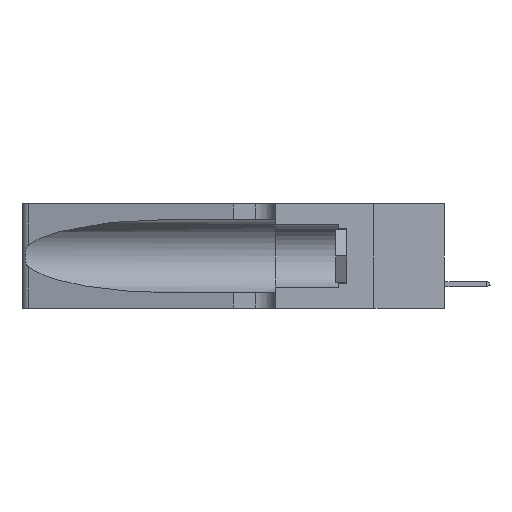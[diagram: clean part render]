
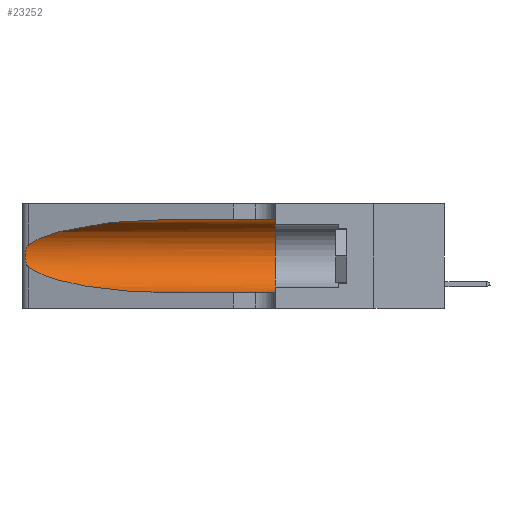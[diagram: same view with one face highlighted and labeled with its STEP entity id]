
A CAD part, left-side view. The second image highlights one B-rep face of the part: STEP entity #23252.
In plain terms, the highlighted cylindrical face has radius 3.308 mm (diameter 6.617 mm), a partial arc.
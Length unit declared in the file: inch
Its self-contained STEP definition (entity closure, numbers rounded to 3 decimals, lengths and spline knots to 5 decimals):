
#1957 = VERTEX_POINT ( 'NONE', #3929 ) ;
#2372 = CARTESIAN_POINT ( 'NONE',  ( 0.1305, 0.35, 0.05475 ) ) ;
#2921 = ORIENTED_EDGE ( 'NONE', *, *, #27712, .T. ) ;
#3313 = FACE_OUTER_BOUND ( 'NONE', #23588, .T. ) ;
#3369 = ORIENTED_EDGE ( 'NONE', *, *, #18472, .T. ) ;
#3929 = CARTESIAN_POINT ( 'NONE',  ( 0.1305, 0.35, 0.31525 ) ) ;
#4199 = CARTESIAN_POINT ( 'NONE',  ( 0.26018, 1.23835, 0.19895 ) ) ;
#4342 = CARTESIAN_POINT ( 'NONE',  ( 0.25854, 1.2359, 0.20912 ) ) ;
#6257 =( BOUNDED_CURVE ( )  B_SPLINE_CURVE ( 3, ( #7449, #13688, #25617, #22827 ),
 .UNSPECIFIED., .F., .T. ) 
 B_SPLINE_CURVE_WITH_KNOTS ( ( 4, 4 ),
 ( 3.44316, 4.71239 ),
 .UNSPECIFIED. ) 
 CURVE ( )  GEOMETRIC_REPRESENTATION_ITEM ( )  RATIONAL_B_SPLINE_CURVE ( ( 1., 0.87, 0.87, 1. ) ) 
 REPRESENTATION_ITEM ( '' )  );
#6865 = EDGE_CURVE ( 'NONE', #1957, #12653, #11539, .T. ) ;
#7319 = CARTESIAN_POINT ( 'NONE',  ( 0.26075, 1.23896, 0.178 ) ) ;
#7449 = CARTESIAN_POINT ( 'NONE',  ( 0.25487, 1.22718, 0.14631 ) ) ;
#9013 = CARTESIAN_POINT ( 'NONE',  ( 0.18966, 0.96281, 0.31525 ) ) ;
#10514 = CARTESIAN_POINT ( 'NONE',  ( 0.26017, 1.23833, 0.17102 ) ) ;
#10752 = AXIS2_PLACEMENT_3D ( 'NONE', #39340, #15642, #24640 ) ;
#11539 = CIRCLE ( 'NONE', #10752, 0.13025 ) ;
#12653 = VERTEX_POINT ( 'NONE', #2372 ) ;
#12994 = CARTESIAN_POINT ( 'NONE',  ( 0.25639, 1.23186, 0.15144 ) ) ;
#13022 = ORIENTED_EDGE ( 'NONE', *, *, #35132, .T. ) ;
#13285 = CARTESIAN_POINT ( 'NONE',  ( 0.25487, 1.22718, 0.22369 ) ) ;
#13558 = VECTOR ( 'NONE', #33225, 39.37008 ) ;
#13688 = CARTESIAN_POINT ( 'NONE',  ( 0.2373, 1.15595, 0.08982 ) ) ;
#14195 = ORIENTED_EDGE ( 'NONE', *, *, #28770, .F. ) ;
#15642 = DIRECTION ( 'NONE',  ( 0., 1., 0. ) ) ;
#15661 = CARTESIAN_POINT ( 'NONE',  ( 0.25487, 1.22718, 0.22369 ) ) ;
#15803 = EDGE_CURVE ( 'NONE', #21686, #26965, #26982, .T. ) ;
#16623 = CARTESIAN_POINT ( 'NONE',  ( 0.25856, 1.23593, 0.16098 ) ) ;
#17494 = CARTESIAN_POINT ( 'NONE',  ( 0.25487, 1.22718, 0.14631 ) ) ;
#18472 = EDGE_CURVE ( 'NONE', #30778, #21686, #22819, .T. ) ;
#19003 = CARTESIAN_POINT ( 'NONE',  ( 0.1305, 0.72297, 0.31525 ) ) ;
#19598 = VECTOR ( 'NONE', #36843, 39.37008 ) ;
#20057 = ORIENTED_EDGE ( 'NONE', *, *, #6865, .F. ) ;
#20108 = VERTEX_POINT ( 'NONE', #27556 ) ;
#21488 = CARTESIAN_POINT ( 'NONE',  ( 0.1305, 1.61858, 0.05475 ) ) ;
#21679 = DIRECTION ( 'NONE',  ( 0., -1., 0. ) ) ;
#21686 = VERTEX_POINT ( 'NONE', #15661 ) ;
#21941 = DIRECTION ( 'NONE',  ( 0., 0., -1. ) ) ;
#22093 = CARTESIAN_POINT ( 'NONE',  ( 0.1305, 1.61858, 0.31525 ) ) ;
#22418 = CARTESIAN_POINT ( 'NONE',  ( 0.25555, 1.22994, 0.2215 ) ) ;
#22689 = CARTESIAN_POINT ( 'NONE',  ( 0.25789, 1.23486, 0.15765 ) ) ;
#22819 =( BOUNDED_CURVE ( )  B_SPLINE_CURVE ( 3, ( #19003, #9013, #37466, #25812 ),
 .UNSPECIFIED., .F., .T. ) 
 B_SPLINE_CURVE_WITH_KNOTS ( ( 4, 4 ),
 ( 1.5708, 2.84003 ),
 .UNSPECIFIED. ) 
 CURVE ( )  GEOMETRIC_REPRESENTATION_ITEM ( )  RATIONAL_B_SPLINE_CURVE ( ( 1., 0.87, 0.87, 1. ) ) 
 REPRESENTATION_ITEM ( '' )  );
#22827 = CARTESIAN_POINT ( 'NONE',  ( 0.1305, 0.72297, 0.05475 ) ) ;
#23252 = ADVANCED_FACE ( 'NONE', ( #3313 ), #35245, .F. ) ;
#23588 = EDGE_LOOP ( 'NONE', ( #3369, #33973, #2921, #13022, #20057, #14195 ) ) ;
#24640 = DIRECTION ( 'NONE',  ( 0., 0., 1. ) ) ;
#25483 = CARTESIAN_POINT ( 'NONE',  ( 0.26075, 1.23896, 0.19203 ) ) ;
#25617 = CARTESIAN_POINT ( 'NONE',  ( 0.18966, 0.96281, 0.05475 ) ) ;
#25812 = CARTESIAN_POINT ( 'NONE',  ( 0.25487, 1.22718, 0.22369 ) ) ;
#25994 = AXIS2_PLACEMENT_3D ( 'NONE', #34018, #21679, #21941 ) ;
#26965 = VERTEX_POINT ( 'NONE', #17494 ) ;
#26982 = B_SPLINE_CURVE_WITH_KNOTS ( 'NONE', 3,
 ( #13285, #22418, #31154, #34498, #4342, #4199, #25483, #7319, #10514, #16623, #22689, #12994, #29345, #38137 ),
 .UNSPECIFIED., .F., .F.,
 ( 4, 2, 2, 2, 2, 2, 4 ),
 ( 0., 0.00027, 0.00053, 0.00107, 0.0016, 0.00187, 0.00214 ),
 .UNSPECIFIED. ) ;
#27556 = CARTESIAN_POINT ( 'NONE',  ( 0.1305, 0.72297, 0.05475 ) ) ;
#27712 = EDGE_CURVE ( 'NONE', #26965, #20108, #6257, .T. ) ;
#27727 = LINE ( 'NONE', #21488, #13558 ) ;
#28585 = LINE ( 'NONE', #22093, #19598 ) ;
#28770 = EDGE_CURVE ( 'NONE', #30778, #1957, #28585, .T. ) ;
#29345 = CARTESIAN_POINT ( 'NONE',  ( 0.25555, 1.22993, 0.14849 ) ) ;
#29881 = CARTESIAN_POINT ( 'NONE',  ( 0.1305, 0.72297, 0.31525 ) ) ;
#30778 = VERTEX_POINT ( 'NONE', #29881 ) ;
#31154 = CARTESIAN_POINT ( 'NONE',  ( 0.25639, 1.23184, 0.21858 ) ) ;
#33225 = DIRECTION ( 'NONE',  ( 0., -1., 0. ) ) ;
#33973 = ORIENTED_EDGE ( 'NONE', *, *, #15803, .T. ) ;
#34018 = CARTESIAN_POINT ( 'NONE',  ( 0.1305, 1.61858, 0.185 ) ) ;
#34498 = CARTESIAN_POINT ( 'NONE',  ( 0.25787, 1.23484, 0.2124 ) ) ;
#35132 = EDGE_CURVE ( 'NONE', #20108, #12653, #27727, .T. ) ;
#35245 = CYLINDRICAL_SURFACE ( 'NONE', #25994, 0.13025 ) ;
#36843 = DIRECTION ( 'NONE',  ( 0., -1., 0. ) ) ;
#37466 = CARTESIAN_POINT ( 'NONE',  ( 0.2373, 1.15595, 0.28018 ) ) ;
#38137 = CARTESIAN_POINT ( 'NONE',  ( 0.25487, 1.22718, 0.14631 ) ) ;
#39340 = CARTESIAN_POINT ( 'NONE',  ( 0.1305, 0.35, 0.185 ) ) ;
